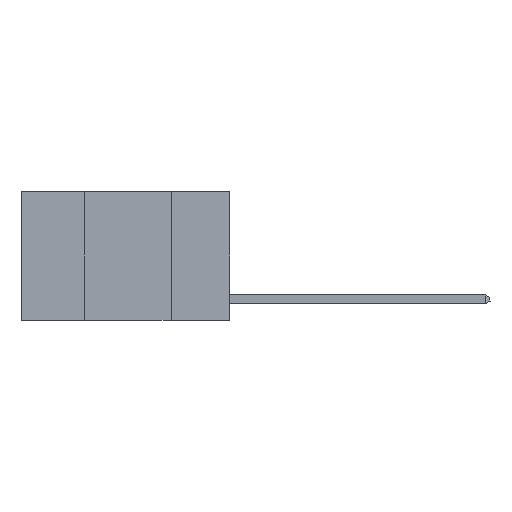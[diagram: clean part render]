
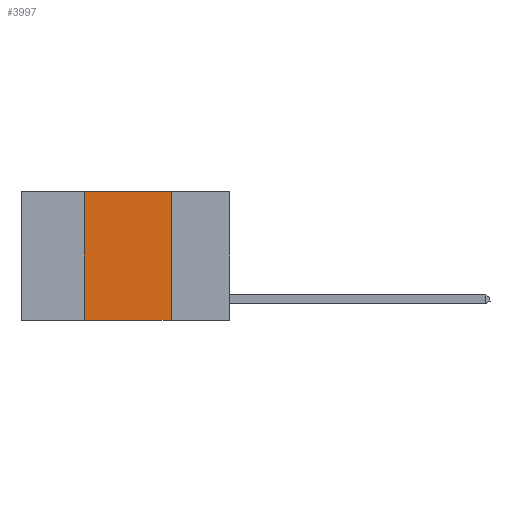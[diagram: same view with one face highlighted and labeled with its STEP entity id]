
A CAD part, left-side view. The second image highlights one B-rep face of the part: STEP entity #3997.
In plain terms, the highlighted planar face has unit normal (-1, 0, 0).
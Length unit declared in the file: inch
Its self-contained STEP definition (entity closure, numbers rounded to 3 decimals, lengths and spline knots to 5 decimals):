
#41 = PLANE ( 'NONE',  #16653 ) ;
#236 = ORIENTED_EDGE ( 'NONE', *, *, #24295, .T. ) ;
#2078 = DIRECTION ( 'NONE',  ( 0., 0., -1. ) ) ;
#2662 = DIRECTION ( 'NONE',  ( 0., 0., 1. ) ) ;
#3224 = ORIENTED_EDGE ( 'NONE', *, *, #19637, .F. ) ;
#3997 = ADVANCED_FACE ( 'NONE', ( #14898 ), #41, .F. ) ;
#4326 = DIRECTION ( 'NONE',  ( 0., 0., -1. ) ) ;
#5503 = CARTESIAN_POINT ( 'NONE',  ( 0., 0.17, -0.37 ) ) ;
#5633 = CARTESIAN_POINT ( 'NONE',  ( 0., 0.42, 0. ) ) ;
#6748 = CARTESIAN_POINT ( 'NONE',  ( 0., 0.17, 0. ) ) ;
#6892 = CARTESIAN_POINT ( 'NONE',  ( 0., 0.42, 0. ) ) ;
#8083 = EDGE_LOOP ( 'NONE', ( #14370, #18330, #3224, #236 ) ) ;
#8361 = CARTESIAN_POINT ( 'NONE',  ( 0., 0.6, -0.37 ) ) ;
#8876 = CARTESIAN_POINT ( 'NONE',  ( 0., 0.6, 0. ) ) ;
#9994 = LINE ( 'NONE', #8876, #26266 ) ;
#10467 = DIRECTION ( 'NONE',  ( 0., -1., 0. ) ) ;
#12564 = CARTESIAN_POINT ( 'NONE',  ( 0., 0.17, 0. ) ) ;
#14370 = ORIENTED_EDGE ( 'NONE', *, *, #26766, .F. ) ;
#14644 = EDGE_CURVE ( 'NONE', #15126, #18957, #9994, .T. ) ;
#14817 = CARTESIAN_POINT ( 'NONE',  ( 0., 0.6, 0. ) ) ;
#14898 = FACE_OUTER_BOUND ( 'NONE', #8083, .T. ) ;
#15126 = VERTEX_POINT ( 'NONE', #5633 ) ;
#16653 = AXIS2_PLACEMENT_3D ( 'NONE', #14817, #16950, #4326 ) ;
#16928 = CARTESIAN_POINT ( 'NONE',  ( 0., 0.42, -0.37 ) ) ;
#16950 = DIRECTION ( 'NONE',  ( 1., 0., 0. ) ) ;
#18330 = ORIENTED_EDGE ( 'NONE', *, *, #14644, .F. ) ;
#18957 = VERTEX_POINT ( 'NONE', #6748 ) ;
#19637 = EDGE_CURVE ( 'NONE', #24873, #15126, #26675, .T. ) ;
#21579 = DIRECTION ( 'NONE',  ( 0., -1., 0. ) ) ;
#22314 = VECTOR ( 'NONE', #10467, 39.37008 ) ;
#22975 = LINE ( 'NONE', #8361, #22314 ) ;
#24295 = EDGE_CURVE ( 'NONE', #24873, #24623, #22975, .T. ) ;
#24623 = VERTEX_POINT ( 'NONE', #5503 ) ;
#24873 = VERTEX_POINT ( 'NONE', #16928 ) ;
#25129 = VECTOR ( 'NONE', #2078, 39.37008 ) ;
#25793 = LINE ( 'NONE', #12564, #25129 ) ;
#26047 = VECTOR ( 'NONE', #2662, 39.37008 ) ;
#26266 = VECTOR ( 'NONE', #21579, 39.37008 ) ;
#26675 = LINE ( 'NONE', #6892, #26047 ) ;
#26766 = EDGE_CURVE ( 'NONE', #18957, #24623, #25793, .T. ) ;
